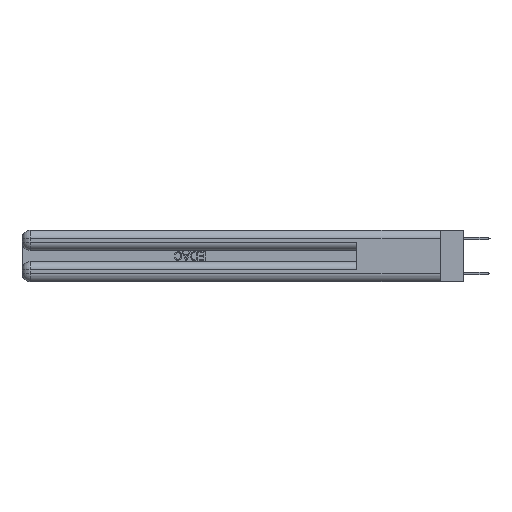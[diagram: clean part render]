
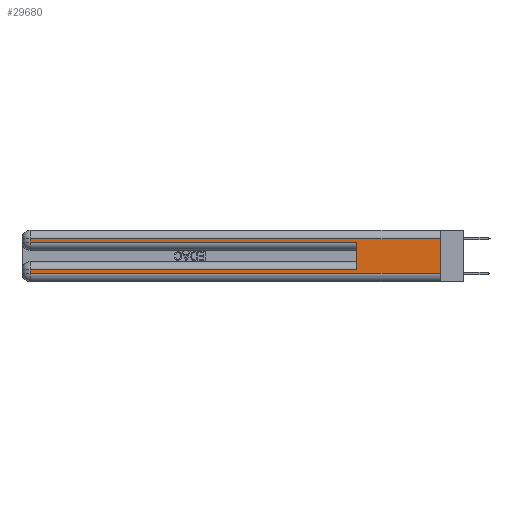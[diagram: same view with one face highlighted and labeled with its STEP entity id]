
A CAD part, left-side view. The second image highlights one B-rep face of the part: STEP entity #29680.
In plain terms, the highlighted planar face has unit normal (-1, 0, 0).
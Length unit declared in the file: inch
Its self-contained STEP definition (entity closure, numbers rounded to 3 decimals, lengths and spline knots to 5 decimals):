
#631 = CARTESIAN_POINT ( 'NONE',  ( 0., 0.6, 0.085 ) ) ;
#804 = CARTESIAN_POINT ( 'NONE',  ( 0., 2.94, 0.37 ) ) ;
#1137 = VECTOR ( 'NONE', #3334, 39.37008 ) ;
#1215 = EDGE_CURVE ( 'NONE', #25613, #8708, #12845, .T. ) ;
#1417 = EDGE_CURVE ( 'NONE', #28395, #21252, #32219, .T. ) ;
#1701 = VECTOR ( 'NONE', #30373, 39.37008 ) ;
#2364 = CARTESIAN_POINT ( 'NONE',  ( 0., 2.94, 0.085 ) ) ;
#3334 = DIRECTION ( 'NONE',  ( 0., 0., -1. ) ) ;
#3506 = ORIENTED_EDGE ( 'NONE', *, *, #17545, .T. ) ;
#3845 = CARTESIAN_POINT ( 'NONE',  ( 0., 0.6, 0.285 ) ) ;
#3851 = CARTESIAN_POINT ( 'NONE',  ( 0., 2.94, 0.285 ) ) ;
#3974 = VECTOR ( 'NONE', #26376, 39.37008 ) ;
#4238 = CARTESIAN_POINT ( 'NONE',  ( 0., 0., 0.085 ) ) ;
#4781 = AXIS2_PLACEMENT_3D ( 'NONE', #8319, #30764, #15987 ) ;
#5318 = VECTOR ( 'NONE', #21090, 39.37008 ) ;
#6323 = CARTESIAN_POINT ( 'NONE',  ( 0., 0.6, 0.145 ) ) ;
#6577 = EDGE_CURVE ( 'NONE', #25613, #21322, #8974, .T. ) ;
#6767 = DIRECTION ( 'NONE',  ( 0., 1., 0. ) ) ;
#7222 = EDGE_CURVE ( 'NONE', #21252, #21322, #14357, .T. ) ;
#7691 = LINE ( 'NONE', #4238, #13653 ) ;
#8056 = DIRECTION ( 'NONE',  ( 0., -1., 0. ) ) ;
#8169 = VECTOR ( 'NONE', #15739, 39.37008 ) ;
#8319 = CARTESIAN_POINT ( 'NONE',  ( 0., 0., 0.37 ) ) ;
#8708 = VERTEX_POINT ( 'NONE', #13797 ) ;
#8974 = LINE ( 'NONE', #18259, #8169 ) ;
#9873 = VERTEX_POINT ( 'NONE', #3851 ) ;
#10380 = CARTESIAN_POINT ( 'NONE',  ( 0., 0., 0.06 ) ) ;
#11615 = CARTESIAN_POINT ( 'NONE',  ( 0., 2.94, 0.06 ) ) ;
#12444 = VECTOR ( 'NONE', #18430, 39.37008 ) ;
#12845 = LINE ( 'NONE', #21162, #5318 ) ;
#13431 = PLANE ( 'NONE',  #4781 ) ;
#13653 = VECTOR ( 'NONE', #6767, 39.37008 ) ;
#13797 = CARTESIAN_POINT ( 'NONE',  ( 0., 2.94, 0.31 ) ) ;
#14357 = LINE ( 'NONE', #10380, #1701 ) ;
#14607 = LINE ( 'NONE', #804, #1137 ) ;
#15739 = DIRECTION ( 'NONE',  ( 0., 0., -1. ) ) ;
#15987 = DIRECTION ( 'NONE',  ( 0., 0., -1. ) ) ;
#17545 = EDGE_CURVE ( 'NONE', #9873, #19721, #18511, .T. ) ;
#17744 = VECTOR ( 'NONE', #8056, 39.37008 ) ;
#17807 = ORIENTED_EDGE ( 'NONE', *, *, #20613, .F. ) ;
#17808 = CARTESIAN_POINT ( 'NONE',  ( 0., 2.94, 0.37 ) ) ;
#18240 = LINE ( 'NONE', #6323, #3974 ) ;
#18259 = CARTESIAN_POINT ( 'NONE',  ( 0., 0., 0.37 ) ) ;
#18430 = DIRECTION ( 'NONE',  ( 0., 0., -1. ) ) ;
#18511 = LINE ( 'NONE', #20627, #17744 ) ;
#18686 = EDGE_LOOP ( 'NONE', ( #22203, #20509, #30510, #3506, #17807, #30570, #31731, #32018 ) ) ;
#19721 = VERTEX_POINT ( 'NONE', #3845 ) ;
#20231 = VERTEX_POINT ( 'NONE', #631 ) ;
#20509 = ORIENTED_EDGE ( 'NONE', *, *, #1215, .T. ) ;
#20613 = EDGE_CURVE ( 'NONE', #20231, #19721, #18240, .T. ) ;
#20627 = CARTESIAN_POINT ( 'NONE',  ( 0., 0., 0.285 ) ) ;
#21090 = DIRECTION ( 'NONE',  ( 0., 1., 0. ) ) ;
#21162 = CARTESIAN_POINT ( 'NONE',  ( 0., 0., 0.31 ) ) ;
#21252 = VERTEX_POINT ( 'NONE', #11615 ) ;
#21322 = VERTEX_POINT ( 'NONE', #26780 ) ;
#22203 = ORIENTED_EDGE ( 'NONE', *, *, #6577, .F. ) ;
#22965 = CARTESIAN_POINT ( 'NONE',  ( 0., 0., 0.31 ) ) ;
#24311 = EDGE_CURVE ( 'NONE', #20231, #28395, #7691, .T. ) ;
#25613 = VERTEX_POINT ( 'NONE', #22965 ) ;
#26150 = FACE_OUTER_BOUND ( 'NONE', #18686, .T. ) ;
#26376 = DIRECTION ( 'NONE',  ( 0., 0., 1. ) ) ;
#26780 = CARTESIAN_POINT ( 'NONE',  ( 0., 0., 0.06 ) ) ;
#28237 = EDGE_CURVE ( 'NONE', #8708, #9873, #14607, .T. ) ;
#28395 = VERTEX_POINT ( 'NONE', #2364 ) ;
#29680 = ADVANCED_FACE ( 'NONE', ( #26150 ), #13431, .F. ) ;
#30373 = DIRECTION ( 'NONE',  ( 0., -1., 0. ) ) ;
#30510 = ORIENTED_EDGE ( 'NONE', *, *, #28237, .T. ) ;
#30570 = ORIENTED_EDGE ( 'NONE', *, *, #24311, .T. ) ;
#30764 = DIRECTION ( 'NONE',  ( 1., 0., 0. ) ) ;
#31731 = ORIENTED_EDGE ( 'NONE', *, *, #1417, .T. ) ;
#32018 = ORIENTED_EDGE ( 'NONE', *, *, #7222, .T. ) ;
#32219 = LINE ( 'NONE', #17808, #12444 ) ;
